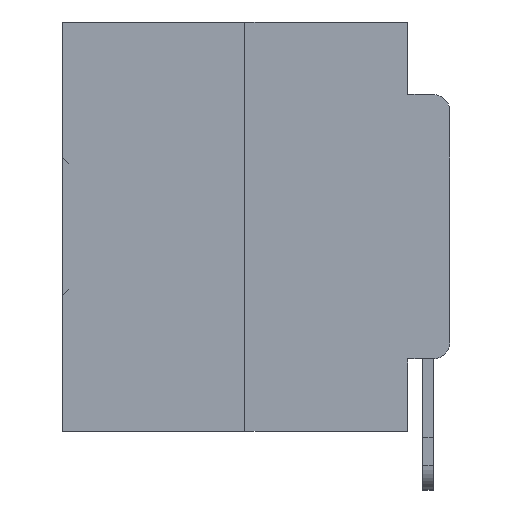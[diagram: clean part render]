
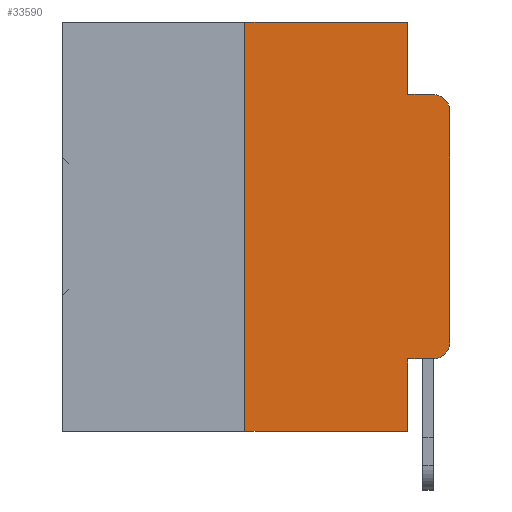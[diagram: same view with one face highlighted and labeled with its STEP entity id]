
A CAD part, left-side view. The second image highlights one B-rep face of the part: STEP entity #33590.
In plain terms, the highlighted planar face has unit normal (-1, 0, 0).
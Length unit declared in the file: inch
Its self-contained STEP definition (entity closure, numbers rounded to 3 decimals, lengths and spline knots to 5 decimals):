
#33 = AXIS2_PLACEMENT_3D ( 'NONE', #26275, #18410, #1801 ) ;
#463 = CARTESIAN_POINT ( 'NONE',  ( 0., 0.473, 0. ) ) ;
#686 = VERTEX_POINT ( 'NONE', #11034 ) ;
#1801 = DIRECTION ( 'NONE',  ( 0., 0., -1. ) ) ;
#1914 = CARTESIAN_POINT ( 'NONE',  ( 0., 0.02, -0.4115 ) ) ;
#2598 = EDGE_CURVE ( 'NONE', #6297, #13085, #28055, .T. ) ;
#2602 = ORIENTED_EDGE ( 'NONE', *, *, #28127, .T. ) ;
#2876 = CARTESIAN_POINT ( 'NONE',  ( 0., 0.051, -0.0885 ) ) ;
#2916 = CARTESIAN_POINT ( 'NONE',  ( 0., 0.051, 0. ) ) ;
#3028 = ORIENTED_EDGE ( 'NONE', *, *, #33473, .T. ) ;
#3698 = FACE_OUTER_BOUND ( 'NONE', #33683, .T. ) ;
#4028 = CARTESIAN_POINT ( 'NONE',  ( 0., 0.051, 0. ) ) ;
#4582 = DIRECTION ( 'NONE',  ( -1., 0., 0. ) ) ;
#6250 = EDGE_CURVE ( 'NONE', #17820, #12876, #27443, .T. ) ;
#6297 = VERTEX_POINT ( 'NONE', #24988 ) ;
#6670 = ORIENTED_EDGE ( 'NONE', *, *, #33692, .T. ) ;
#6730 = VERTEX_POINT ( 'NONE', #11143 ) ;
#7316 = VERTEX_POINT ( 'NONE', #24038 ) ;
#7618 = VECTOR ( 'NONE', #7784, 39.37008 ) ;
#7636 = EDGE_CURVE ( 'NONE', #686, #6730, #12102, .T. ) ;
#7784 = DIRECTION ( 'NONE',  ( 0., -1., 0. ) ) ;
#8074 = LINE ( 'NONE', #28562, #35112 ) ;
#8790 = EDGE_CURVE ( 'NONE', #27467, #6297, #30873, .T. ) ;
#9176 = CIRCLE ( 'NONE', #34823, 0.02 ) ;
#10093 = VERTEX_POINT ( 'NONE', #30802 ) ;
#10428 = ORIENTED_EDGE ( 'NONE', *, *, #6250, .F. ) ;
#11034 = CARTESIAN_POINT ( 'NONE',  ( 0., 0.051, -0.4115 ) ) ;
#11143 = CARTESIAN_POINT ( 'NONE',  ( 0., 0.051, -0.5 ) ) ;
#11411 = DIRECTION ( 'NONE',  ( 0., -1., 0. ) ) ;
#11498 = DIRECTION ( 'NONE',  ( -1., 0., 0. ) ) ;
#11661 = DIRECTION ( 'NONE',  ( 0., -1., 0. ) ) ;
#11978 = VECTOR ( 'NONE', #27801, 39.37008 ) ;
#12102 = LINE ( 'NONE', #25504, #18541 ) ;
#12876 = VERTEX_POINT ( 'NONE', #27760 ) ;
#13085 = VERTEX_POINT ( 'NONE', #4028 ) ;
#13758 = VECTOR ( 'NONE', #16748, 39.37008 ) ;
#14713 = DIRECTION ( 'NONE',  ( 0., 0., 1. ) ) ;
#15002 = LINE ( 'NONE', #18752, #7618 ) ;
#15761 = EDGE_CURVE ( 'NONE', #27829, #7316, #9176, .T. ) ;
#16661 = VECTOR ( 'NONE', #14713, 39.37008 ) ;
#16748 = DIRECTION ( 'NONE',  ( 0., 0., -1. ) ) ;
#16879 = CARTESIAN_POINT ( 'NONE',  ( 0., 0.25, -0.5 ) ) ;
#17413 = DIRECTION ( 'NONE',  ( 0., 0., -1. ) ) ;
#17466 = CARTESIAN_POINT ( 'NONE',  ( 0., 0.25, 0. ) ) ;
#17820 = VERTEX_POINT ( 'NONE', #2876 ) ;
#18410 = DIRECTION ( 'NONE',  ( 1., 0., 0. ) ) ;
#18541 = VECTOR ( 'NONE', #17413, 39.37008 ) ;
#18752 = CARTESIAN_POINT ( 'NONE',  ( 0., 0.051, -0.4115 ) ) ;
#19492 = VECTOR ( 'NONE', #11411, 39.37008 ) ;
#20391 = ORIENTED_EDGE ( 'NONE', *, *, #27567, .T. ) ;
#20737 = VECTOR ( 'NONE', #11661, 39.37008 ) ;
#21056 = CARTESIAN_POINT ( 'NONE',  ( 0., 0.02, -0.3915 ) ) ;
#22167 = CARTESIAN_POINT ( 'NONE',  ( 0., 0.051, -0.0885 ) ) ;
#23778 = DIRECTION ( 'NONE',  ( 0., 0., -1. ) ) ;
#24038 = CARTESIAN_POINT ( 'NONE',  ( 0., 0., -0.3915 ) ) ;
#24988 = CARTESIAN_POINT ( 'NONE',  ( 0., 0.25, 0. ) ) ;
#25504 = CARTESIAN_POINT ( 'NONE',  ( 0., 0.051, 0. ) ) ;
#26275 = CARTESIAN_POINT ( 'NONE',  ( 0., 0.473, 0. ) ) ;
#27149 = ORIENTED_EDGE ( 'NONE', *, *, #15761, .T. ) ;
#27443 = LINE ( 'NONE', #22167, #19492 ) ;
#27467 = VERTEX_POINT ( 'NONE', #16879 ) ;
#27567 = EDGE_CURVE ( 'NONE', #27467, #6730, #34910, .T. ) ;
#27723 = CARTESIAN_POINT ( 'NONE',  ( 0., 0.02, -0.1085 ) ) ;
#27760 = CARTESIAN_POINT ( 'NONE',  ( 0., 0.02, -0.0885 ) ) ;
#27801 = DIRECTION ( 'NONE',  ( 0., -1., 0. ) ) ;
#27829 = VERTEX_POINT ( 'NONE', #1914 ) ;
#27924 = ORIENTED_EDGE ( 'NONE', *, *, #7636, .F. ) ;
#28055 = LINE ( 'NONE', #463, #11978 ) ;
#28127 = EDGE_CURVE ( 'NONE', #10093, #12876, #33184, .T. ) ;
#28562 = CARTESIAN_POINT ( 'NONE',  ( 0., 0., 0. ) ) ;
#29021 = PLANE ( 'NONE',  #33 ) ;
#29695 = AXIS2_PLACEMENT_3D ( 'NONE', #27723, #11498, #30392 ) ;
#30392 = DIRECTION ( 'NONE',  ( 0., 0., -1. ) ) ;
#30802 = CARTESIAN_POINT ( 'NONE',  ( 0., 0., -0.1085 ) ) ;
#30873 = LINE ( 'NONE', #17466, #16661 ) ;
#31251 = DIRECTION ( 'NONE',  ( 0., 0., 1. ) ) ;
#32342 = EDGE_CURVE ( 'NONE', #13085, #17820, #35139, .T. ) ;
#32859 = ORIENTED_EDGE ( 'NONE', *, *, #2598, .F. ) ;
#33184 = CIRCLE ( 'NONE', #29695, 0.02 ) ;
#33221 = CARTESIAN_POINT ( 'NONE',  ( 0., 0.473, -0.5 ) ) ;
#33256 = ORIENTED_EDGE ( 'NONE', *, *, #32342, .F. ) ;
#33291 = ORIENTED_EDGE ( 'NONE', *, *, #8790, .F. ) ;
#33473 = EDGE_CURVE ( 'NONE', #7316, #10093, #8074, .T. ) ;
#33590 = ADVANCED_FACE ( 'NONE', ( #3698 ), #29021, .F. ) ;
#33683 = EDGE_LOOP ( 'NONE', ( #3028, #2602, #10428, #33256, #32859, #33291, #20391, #27924, #6670, #27149 ) ) ;
#33692 = EDGE_CURVE ( 'NONE', #686, #27829, #15002, .T. ) ;
#34823 = AXIS2_PLACEMENT_3D ( 'NONE', #21056, #4582, #23778 ) ;
#34910 = LINE ( 'NONE', #33221, #20737 ) ;
#35112 = VECTOR ( 'NONE', #31251, 39.37008 ) ;
#35139 = LINE ( 'NONE', #2916, #13758 ) ;
